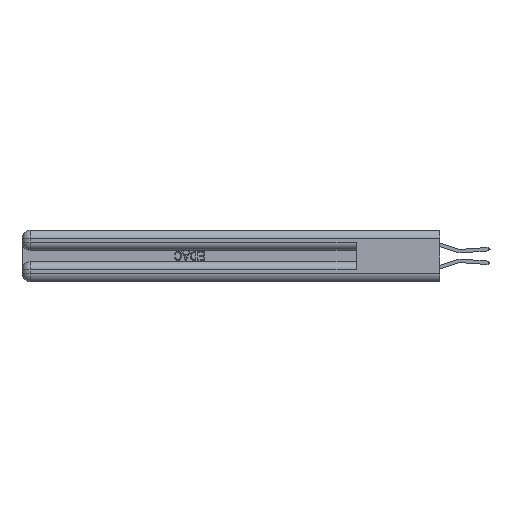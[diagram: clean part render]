
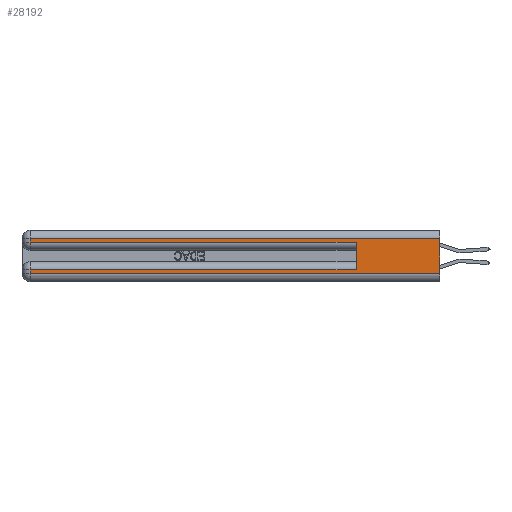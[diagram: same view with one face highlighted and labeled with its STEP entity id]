
A CAD part, left-side view. The second image highlights one B-rep face of the part: STEP entity #28192.
In plain terms, the highlighted planar face has unit normal (-1, 0, 0).
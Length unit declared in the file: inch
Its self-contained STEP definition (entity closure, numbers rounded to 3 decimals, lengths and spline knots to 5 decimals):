
#1517 = VECTOR ( 'NONE', #39855, 39.37008 ) ;
#1902 = LINE ( 'NONE', #36634, #40251 ) ;
#2009 = VECTOR ( 'NONE', #42217, 39.37008 ) ;
#2158 = EDGE_CURVE ( 'NONE', #14206, #2456, #39317, .T. ) ;
#2456 = VERTEX_POINT ( 'NONE', #39191 ) ;
#3143 = CARTESIAN_POINT ( 'NONE',  ( 0., 0., 0.37 ) ) ;
#3202 = EDGE_CURVE ( 'NONE', #11904, #12482, #1902, .T. ) ;
#3321 = VERTEX_POINT ( 'NONE', #8134 ) ;
#3888 = ORIENTED_EDGE ( 'NONE', *, *, #18616, .T. ) ;
#3964 = ORIENTED_EDGE ( 'NONE', *, *, #3202, .T. ) ;
#6964 = ORIENTED_EDGE ( 'NONE', *, *, #19065, .F. ) ;
#7913 = DIRECTION ( 'NONE',  ( 0., -1., 0. ) ) ;
#8029 = CARTESIAN_POINT ( 'NONE',  ( 0., 0., 0.37 ) ) ;
#8134 = CARTESIAN_POINT ( 'NONE',  ( 0., 0., 0.06 ) ) ;
#8146 = ORIENTED_EDGE ( 'NONE', *, *, #15304, .F. ) ;
#8285 = CARTESIAN_POINT ( 'NONE',  ( 0., 2.94, 0.31 ) ) ;
#10682 = PLANE ( 'NONE',  #40683 ) ;
#10958 = LINE ( 'NONE', #17614, #44050 ) ;
#11635 = DIRECTION ( 'NONE',  ( 1., 0., 0. ) ) ;
#11904 = VERTEX_POINT ( 'NONE', #28406 ) ;
#12482 = VERTEX_POINT ( 'NONE', #32137 ) ;
#13081 = FACE_OUTER_BOUND ( 'NONE', #26310, .T. ) ;
#13155 = DIRECTION ( 'NONE',  ( 0., 0., 1. ) ) ;
#14206 = VERTEX_POINT ( 'NONE', #27995 ) ;
#14386 = DIRECTION ( 'NONE',  ( 0., 0., -1. ) ) ;
#15304 = EDGE_CURVE ( 'NONE', #43630, #3321, #30988, .T. ) ;
#15718 = CARTESIAN_POINT ( 'NONE',  ( 0., 0.6, 0.085 ) ) ;
#17614 = CARTESIAN_POINT ( 'NONE',  ( 0., 0., 0.06 ) ) ;
#18616 = EDGE_CURVE ( 'NONE', #23615, #11904, #40892, .T. ) ;
#19065 = EDGE_CURVE ( 'NONE', #23615, #2456, #29684, .T. ) ;
#19600 = LINE ( 'NONE', #22873, #1517 ) ;
#21965 = VECTOR ( 'NONE', #26521, 39.37008 ) ;
#22406 = EDGE_CURVE ( 'NONE', #12482, #3321, #10958, .T. ) ;
#22873 = CARTESIAN_POINT ( 'NONE',  ( 0., 0., 0.31 ) ) ;
#23615 = VERTEX_POINT ( 'NONE', #15718 ) ;
#25403 = VECTOR ( 'NONE', #13155, 39.37008 ) ;
#26310 = EDGE_LOOP ( 'NONE', ( #8146, #30677, #33488, #42450, #6964, #3888, #3964, #36516 ) ) ;
#26521 = DIRECTION ( 'NONE',  ( 0., 0., -1. ) ) ;
#27151 = VECTOR ( 'NONE', #14386, 39.37008 ) ;
#27995 = CARTESIAN_POINT ( 'NONE',  ( 0., 2.94, 0.285 ) ) ;
#28192 = ADVANCED_FACE ( 'NONE', ( #13081 ), #10682, .F. ) ;
#28406 = CARTESIAN_POINT ( 'NONE',  ( 0., 2.94, 0.085 ) ) ;
#28601 = CARTESIAN_POINT ( 'NONE',  ( 0., 0.6, 0.145 ) ) ;
#28913 = DIRECTION ( 'NONE',  ( 0., 0., -1. ) ) ;
#29161 = VECTOR ( 'NONE', #42862, 39.37008 ) ;
#29684 = LINE ( 'NONE', #28601, #25403 ) ;
#30677 = ORIENTED_EDGE ( 'NONE', *, *, #37854, .T. ) ;
#30988 = LINE ( 'NONE', #3143, #21965 ) ;
#32137 = CARTESIAN_POINT ( 'NONE',  ( 0., 2.94, 0.06 ) ) ;
#33021 = LINE ( 'NONE', #38683, #27151 ) ;
#33262 = VERTEX_POINT ( 'NONE', #8285 ) ;
#33488 = ORIENTED_EDGE ( 'NONE', *, *, #41673, .T. ) ;
#33600 = CARTESIAN_POINT ( 'NONE',  ( 0., 0., 0.31 ) ) ;
#36350 = DIRECTION ( 'NONE',  ( 0., 0., -1. ) ) ;
#36516 = ORIENTED_EDGE ( 'NONE', *, *, #22406, .T. ) ;
#36634 = CARTESIAN_POINT ( 'NONE',  ( 0., 2.94, 0.37 ) ) ;
#37854 = EDGE_CURVE ( 'NONE', #43630, #33262, #19600, .T. ) ;
#38683 = CARTESIAN_POINT ( 'NONE',  ( 0., 2.94, 0.37 ) ) ;
#39191 = CARTESIAN_POINT ( 'NONE',  ( 0., 0.6, 0.285 ) ) ;
#39317 = LINE ( 'NONE', #43451, #29161 ) ;
#39855 = DIRECTION ( 'NONE',  ( 0., 1., 0. ) ) ;
#40251 = VECTOR ( 'NONE', #36350, 39.37008 ) ;
#40683 = AXIS2_PLACEMENT_3D ( 'NONE', #8029, #11635, #28913 ) ;
#40892 = LINE ( 'NONE', #42668, #2009 ) ;
#41673 = EDGE_CURVE ( 'NONE', #33262, #14206, #33021, .T. ) ;
#42217 = DIRECTION ( 'NONE',  ( 0., 1., 0. ) ) ;
#42450 = ORIENTED_EDGE ( 'NONE', *, *, #2158, .T. ) ;
#42668 = CARTESIAN_POINT ( 'NONE',  ( 0., 0., 0.085 ) ) ;
#42862 = DIRECTION ( 'NONE',  ( 0., -1., 0. ) ) ;
#43451 = CARTESIAN_POINT ( 'NONE',  ( 0., 0., 0.285 ) ) ;
#43630 = VERTEX_POINT ( 'NONE', #33600 ) ;
#44050 = VECTOR ( 'NONE', #7913, 39.37008 ) ;
